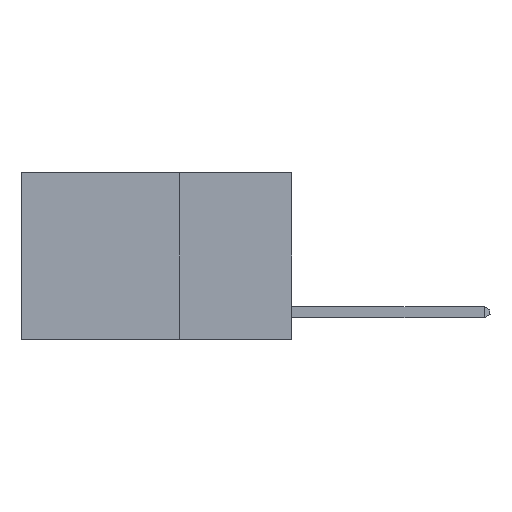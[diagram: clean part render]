
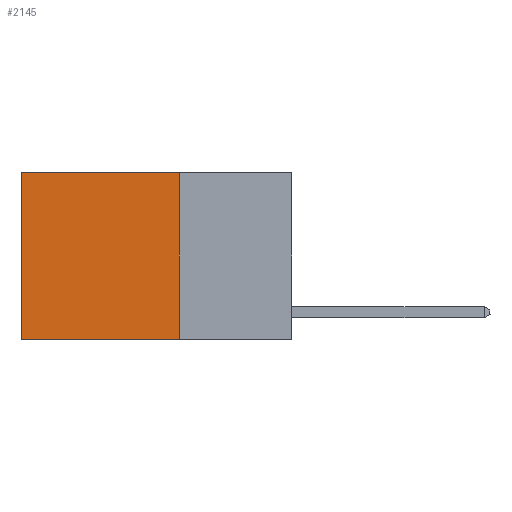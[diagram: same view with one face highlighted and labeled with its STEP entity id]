
A CAD part, left-side view. The second image highlights one B-rep face of the part: STEP entity #2145.
In plain terms, the highlighted planar face has unit normal (-1, 0, 0).
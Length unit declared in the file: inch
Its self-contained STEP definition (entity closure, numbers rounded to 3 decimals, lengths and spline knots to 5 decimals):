
#259 = DIRECTION ( 'NONE',  ( 0., 1., 0. ) ) ;
#346 = CARTESIAN_POINT ( 'NONE',  ( 0.2625, 0.25, 0. ) ) ;
#876 = EDGE_CURVE ( 'NONE', #6358, #4630, #8932, .T. ) ;
#1149 = CARTESIAN_POINT ( 'NONE',  ( 0.2625, 0.6, -0.37 ) ) ;
#1379 = CARTESIAN_POINT ( 'NONE',  ( 0.2625, 0.25, 0. ) ) ;
#1414 = LINE ( 'NONE', #8027, #4643 ) ;
#1501 = CARTESIAN_POINT ( 'NONE',  ( 0.2625, 0.25, 0. ) ) ;
#2040 = VECTOR ( 'NONE', #3086, 39.37008 ) ;
#2145 = ADVANCED_FACE ( 'NONE', ( #3378 ), #5262, .F. ) ;
#2799 = ORIENTED_EDGE ( 'NONE', *, *, #6126, .T. ) ;
#2917 = ORIENTED_EDGE ( 'NONE', *, *, #12279, .F. ) ;
#3086 = DIRECTION ( 'NONE',  ( 0., 0., -1. ) ) ;
#3317 = VECTOR ( 'NONE', #11946, 39.37008 ) ;
#3378 = FACE_OUTER_BOUND ( 'NONE', #9403, .T. ) ;
#3412 = VERTEX_POINT ( 'NONE', #1149 ) ;
#3461 = ORIENTED_EDGE ( 'NONE', *, *, #7749, .F. ) ;
#4630 = VERTEX_POINT ( 'NONE', #7259 ) ;
#4643 = VECTOR ( 'NONE', #9032, 39.37008 ) ;
#5197 = DIRECTION ( 'NONE',  ( 0., 0., -1. ) ) ;
#5262 = PLANE ( 'NONE',  #6458 ) ;
#5321 = VERTEX_POINT ( 'NONE', #12137 ) ;
#6126 = EDGE_CURVE ( 'NONE', #4630, #3412, #1414, .T. ) ;
#6326 = CARTESIAN_POINT ( 'NONE',  ( 0.2625, 0.25, 0. ) ) ;
#6343 = LINE ( 'NONE', #9297, #3317 ) ;
#6358 = VERTEX_POINT ( 'NONE', #6326 ) ;
#6458 = AXIS2_PLACEMENT_3D ( 'NONE', #1501, #8933, #5197 ) ;
#7259 = CARTESIAN_POINT ( 'NONE',  ( 0.2625, 0.6, 0. ) ) ;
#7749 = EDGE_CURVE ( 'NONE', #6358, #5321, #11831, .T. ) ;
#8027 = CARTESIAN_POINT ( 'NONE',  ( 0.2625, 0.6, 0. ) ) ;
#8613 = ORIENTED_EDGE ( 'NONE', *, *, #876, .T. ) ;
#8932 = LINE ( 'NONE', #1379, #9195 ) ;
#8933 = DIRECTION ( 'NONE',  ( 1., 0., 0. ) ) ;
#9032 = DIRECTION ( 'NONE',  ( 0., 0., -1. ) ) ;
#9195 = VECTOR ( 'NONE', #259, 39.37008 ) ;
#9297 = CARTESIAN_POINT ( 'NONE',  ( 0.2625, 0.25, -0.37 ) ) ;
#9403 = EDGE_LOOP ( 'NONE', ( #2799, #2917, #3461, #8613 ) ) ;
#11831 = LINE ( 'NONE', #346, #2040 ) ;
#11946 = DIRECTION ( 'NONE',  ( 0., 1., 0. ) ) ;
#12137 = CARTESIAN_POINT ( 'NONE',  ( 0.2625, 0.25, -0.37 ) ) ;
#12279 = EDGE_CURVE ( 'NONE', #5321, #3412, #6343, .T. ) ;
